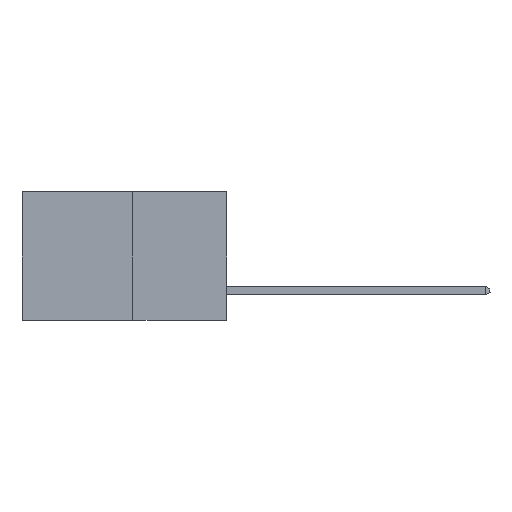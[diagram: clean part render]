
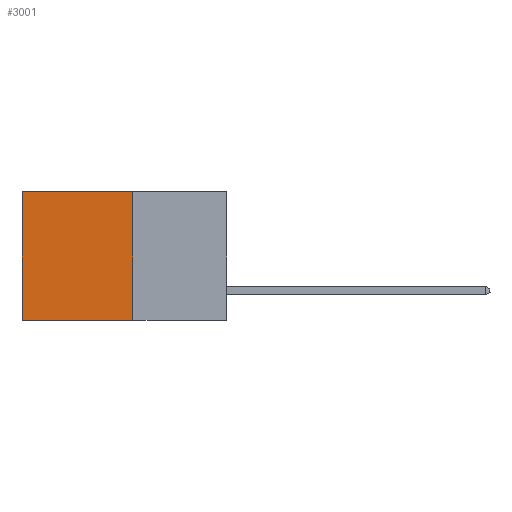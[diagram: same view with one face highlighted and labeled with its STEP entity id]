
A CAD part, left-side view. The second image highlights one B-rep face of the part: STEP entity #3001.
In plain terms, the highlighted planar face has unit normal (-1, 0, 0).
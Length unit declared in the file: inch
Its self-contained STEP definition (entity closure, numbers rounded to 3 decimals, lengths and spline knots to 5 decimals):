
#685 = DIRECTION ( 'NONE',  ( 0., 1., 0. ) ) ;
#764 = VERTEX_POINT ( 'NONE', #5904 ) ;
#822 = DIRECTION ( 'NONE',  ( 0., 0., -1. ) ) ;
#1217 = VERTEX_POINT ( 'NONE', #14789 ) ;
#1608 = LINE ( 'NONE', #22124, #10692 ) ;
#1716 = CARTESIAN_POINT ( 'NONE',  ( 0.277, 0.27, -0.37 ) ) ;
#1996 = ORIENTED_EDGE ( 'NONE', *, *, #14626, .T. ) ;
#2295 = LINE ( 'NONE', #4276, #6582 ) ;
#3001 = ADVANCED_FACE ( 'NONE', ( #7291 ), #16247, .F. ) ;
#4276 = CARTESIAN_POINT ( 'NONE',  ( 0.277, 0.27, 0. ) ) ;
#5586 = EDGE_CURVE ( 'NONE', #11007, #22137, #8053, .T. ) ;
#5904 = CARTESIAN_POINT ( 'NONE',  ( 0.277, 0.27, 0. ) ) ;
#6106 = DIRECTION ( 'NONE',  ( 0., 1., 0. ) ) ;
#6582 = VECTOR ( 'NONE', #6106, 39.37008 ) ;
#7291 = FACE_OUTER_BOUND ( 'NONE', #15918, .T. ) ;
#8053 = LINE ( 'NONE', #20465, #21594 ) ;
#9681 = AXIS2_PLACEMENT_3D ( 'NONE', #1716, #14153, #15047 ) ;
#10190 = CARTESIAN_POINT ( 'NONE',  ( 0.277, 0.59, -0.37 ) ) ;
#10692 = VECTOR ( 'NONE', #685, 39.37008 ) ;
#11007 = VERTEX_POINT ( 'NONE', #11399 ) ;
#11399 = CARTESIAN_POINT ( 'NONE',  ( 0.277, 0.59, 0. ) ) ;
#11948 = ORIENTED_EDGE ( 'NONE', *, *, #5586, .T. ) ;
#14153 = DIRECTION ( 'NONE',  ( 1., 0., 0. ) ) ;
#14626 = EDGE_CURVE ( 'NONE', #764, #11007, #2295, .T. ) ;
#14789 = CARTESIAN_POINT ( 'NONE',  ( 0.277, 0.27, -0.37 ) ) ;
#15047 = DIRECTION ( 'NONE',  ( 0., 0., -1. ) ) ;
#15918 = EDGE_LOOP ( 'NONE', ( #11948, #21282, #18862, #1996 ) ) ;
#16247 = PLANE ( 'NONE',  #9681 ) ;
#17011 = CARTESIAN_POINT ( 'NONE',  ( 0.277, 0.27, -0.37 ) ) ;
#17590 = VECTOR ( 'NONE', #822, 39.37008 ) ;
#18141 = LINE ( 'NONE', #17011, #17590 ) ;
#18862 = ORIENTED_EDGE ( 'NONE', *, *, #20499, .F. ) ;
#19413 = EDGE_CURVE ( 'NONE', #1217, #22137, #1608, .T. ) ;
#19954 = DIRECTION ( 'NONE',  ( 0., 0., -1. ) ) ;
#20465 = CARTESIAN_POINT ( 'NONE',  ( 0.277, 0.59, -0.37 ) ) ;
#20499 = EDGE_CURVE ( 'NONE', #764, #1217, #18141, .T. ) ;
#21282 = ORIENTED_EDGE ( 'NONE', *, *, #19413, .F. ) ;
#21594 = VECTOR ( 'NONE', #19954, 39.37008 ) ;
#22124 = CARTESIAN_POINT ( 'NONE',  ( 0.277, 0.27, -0.37 ) ) ;
#22137 = VERTEX_POINT ( 'NONE', #10190 ) ;
